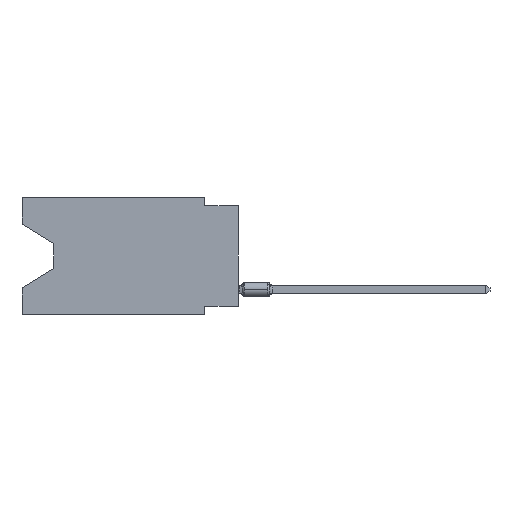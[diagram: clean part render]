
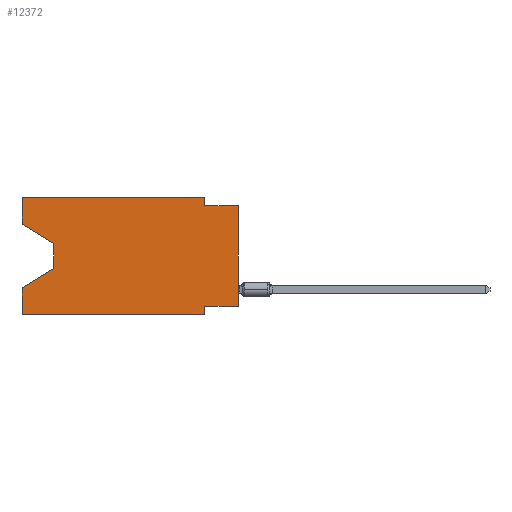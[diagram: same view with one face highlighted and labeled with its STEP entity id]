
A CAD part, left-side view. The second image highlights one B-rep face of the part: STEP entity #12372.
In plain terms, the highlighted planar face has unit normal (-1, 0, 0).
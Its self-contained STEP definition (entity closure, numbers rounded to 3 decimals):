
#201 = VECTOR ( 'NONE', #5137, 1000. ) ;
#222 = AXIS2_PLACEMENT_3D ( 'NONE', #23340, #15614, #23591 ) ;
#711 = ORIENTED_EDGE ( 'NONE', *, *, #15531, .F. ) ;
#891 = ORIENTED_EDGE ( 'NONE', *, *, #18024, .T. ) ;
#923 = CARTESIAN_POINT ( 'NONE',  ( 0., 2.54, 0. ) ) ;
#1017 = VECTOR ( 'NONE', #20075, 1000. ) ;
#1238 = CARTESIAN_POINT ( 'NONE',  ( 0., 16.383, 0. ) ) ;
#1484 = VECTOR ( 'NONE', #4915, 1000. ) ;
#2024 = CARTESIAN_POINT ( 'NONE',  ( 0., 16.383, 0. ) ) ;
#3054 = LINE ( 'NONE', #1238, #4397 ) ;
#3088 = EDGE_CURVE ( 'NONE', #4136, #11339, #17295, .T. ) ;
#3145 = DIRECTION ( 'NONE',  ( 0., 0.855, -0.519 ) ) ;
#3337 = CARTESIAN_POINT ( 'NONE',  ( 0., 13.97, -5.385 ) ) ;
#3357 = LINE ( 'NONE', #13306, #1484 ) ;
#3434 = ORIENTED_EDGE ( 'NONE', *, *, #7880, .F. ) ;
#3718 = EDGE_CURVE ( 'NONE', #4136, #8840, #11868, .T. ) ;
#3720 = CARTESIAN_POINT ( 'NONE',  ( 0., 13.97, -3.505 ) ) ;
#3950 = EDGE_CURVE ( 'NONE', #8452, #16788, #3357, .T. ) ;
#4136 = VERTEX_POINT ( 'NONE', #21675 ) ;
#4397 = VECTOR ( 'NONE', #19028, 1000. ) ;
#4427 = DIRECTION ( 'NONE',  ( 0., -0.855, -0.519 ) ) ;
#4524 = CARTESIAN_POINT ( 'NONE',  ( 0., 16.383, 0. ) ) ;
#4723 = VERTEX_POINT ( 'NONE', #15163 ) ;
#4743 = VECTOR ( 'NONE', #5638, 1000. ) ;
#4868 = VECTOR ( 'NONE', #4427, 1000. ) ;
#4890 = CARTESIAN_POINT ( 'NONE',  ( 0., 0., -0.635 ) ) ;
#4915 = DIRECTION ( 'NONE',  ( 0., 0., -1. ) ) ;
#5137 = DIRECTION ( 'NONE',  ( 0., -1., 0. ) ) ;
#5200 = VECTOR ( 'NONE', #20013, 1000. ) ;
#5401 = FACE_OUTER_BOUND ( 'NONE', #20268, .T. ) ;
#5638 = DIRECTION ( 'NONE',  ( 0., 1., 0. ) ) ;
#6662 = ORIENTED_EDGE ( 'NONE', *, *, #24161, .F. ) ;
#6901 = EDGE_CURVE ( 'NONE', #18964, #8840, #8803, .T. ) ;
#6998 = ORIENTED_EDGE ( 'NONE', *, *, #24707, .F. ) ;
#7002 = VECTOR ( 'NONE', #21537, 1000. ) ;
#7880 = EDGE_CURVE ( 'NONE', #14816, #18964, #18946, .T. ) ;
#8199 = DIRECTION ( 'NONE',  ( 0., 0., -1. ) ) ;
#8452 = VERTEX_POINT ( 'NONE', #3720 ) ;
#8803 = LINE ( 'NONE', #4890, #201 ) ;
#8840 = VERTEX_POINT ( 'NONE', #25519 ) ;
#8968 = VERTEX_POINT ( 'NONE', #10076 ) ;
#10076 = CARTESIAN_POINT ( 'NONE',  ( 0., 16.383, -6.852 ) ) ;
#10216 = ORIENTED_EDGE ( 'NONE', *, *, #3088, .F. ) ;
#10373 = CARTESIAN_POINT ( 'NONE',  ( 0., 16.383, 0. ) ) ;
#10803 = LINE ( 'NONE', #16574, #12685 ) ;
#11339 = VERTEX_POINT ( 'NONE', #22274 ) ;
#11868 = LINE ( 'NONE', #12014, #5200 ) ;
#12014 = CARTESIAN_POINT ( 'NONE',  ( 0., 0., 0. ) ) ;
#12113 = LINE ( 'NONE', #17625, #7002 ) ;
#12372 = ADVANCED_FACE ( 'NONE', ( #5401 ), #23738, .F. ) ;
#12394 = VECTOR ( 'NONE', #3145, 1000. ) ;
#12685 = VECTOR ( 'NONE', #8199, 1000. ) ;
#12788 = ORIENTED_EDGE ( 'NONE', *, *, #25730, .F. ) ;
#13306 = CARTESIAN_POINT ( 'NONE',  ( 0., 13.97, -3.505 ) ) ;
#13551 = ORIENTED_EDGE ( 'NONE', *, *, #14973, .T. ) ;
#14527 = ORIENTED_EDGE ( 'NONE', *, *, #16674, .T. ) ;
#14816 = VERTEX_POINT ( 'NONE', #923 ) ;
#14973 = EDGE_CURVE ( 'NONE', #16788, #8968, #19125, .T. ) ;
#15055 = CARTESIAN_POINT ( 'NONE',  ( 0., 13.97, -5.385 ) ) ;
#15163 = CARTESIAN_POINT ( 'NONE',  ( 0., 16.383, -8.89 ) ) ;
#15531 = EDGE_CURVE ( 'NONE', #11339, #19263, #10803, .T. ) ;
#15614 = DIRECTION ( 'NONE',  ( 1., 0., 0. ) ) ;
#16260 = ORIENTED_EDGE ( 'NONE', *, *, #3718, .T. ) ;
#16574 = CARTESIAN_POINT ( 'NONE',  ( 0., 2.54, -8.89 ) ) ;
#16674 = EDGE_CURVE ( 'NONE', #23670, #8452, #20630, .T. ) ;
#16788 = VERTEX_POINT ( 'NONE', #3337 ) ;
#17295 = LINE ( 'NONE', #21351, #4743 ) ;
#17625 = CARTESIAN_POINT ( 'NONE',  ( 0., 16.383, -8.89 ) ) ;
#18019 = CARTESIAN_POINT ( 'NONE',  ( 0., 2.54, -8.89 ) ) ;
#18024 = EDGE_CURVE ( 'NONE', #4723, #19263, #12113, .T. ) ;
#18239 = LINE ( 'NONE', #2024, #1017 ) ;
#18946 = LINE ( 'NONE', #24976, #25599 ) ;
#18964 = VERTEX_POINT ( 'NONE', #22346 ) ;
#19028 = DIRECTION ( 'NONE',  ( 0., 0., 1. ) ) ;
#19125 = LINE ( 'NONE', #15055, #12394 ) ;
#19263 = VERTEX_POINT ( 'NONE', #18019 ) ;
#19901 = ORIENTED_EDGE ( 'NONE', *, *, #6901, .F. ) ;
#19947 = DIRECTION ( 'NONE',  ( 0., 0., 1. ) ) ;
#20013 = DIRECTION ( 'NONE',  ( 0., 0., 1. ) ) ;
#20075 = DIRECTION ( 'NONE',  ( 0., -1., 0. ) ) ;
#20178 = ORIENTED_EDGE ( 'NONE', *, *, #3950, .T. ) ;
#20190 = LINE ( 'NONE', #10373, #24399 ) ;
#20268 = EDGE_LOOP ( 'NONE', ( #14527, #20178, #13551, #12788, #891, #711, #10216, #16260, #19901, #3434, #6998, #6662 ) ) ;
#20584 = VERTEX_POINT ( 'NONE', #4524 ) ;
#20630 = LINE ( 'NONE', #22347, #4868 ) ;
#21026 = DIRECTION ( 'NONE',  ( 0., 0., -1. ) ) ;
#21174 = CARTESIAN_POINT ( 'NONE',  ( 0., 16.383, -2.038 ) ) ;
#21351 = CARTESIAN_POINT ( 'NONE',  ( 0., 0., -8.255 ) ) ;
#21537 = DIRECTION ( 'NONE',  ( 0., -1., 0. ) ) ;
#21675 = CARTESIAN_POINT ( 'NONE',  ( 0., 0., -8.255 ) ) ;
#22274 = CARTESIAN_POINT ( 'NONE',  ( 0., 2.54, -8.255 ) ) ;
#22346 = CARTESIAN_POINT ( 'NONE',  ( 0., 2.54, -0.635 ) ) ;
#22347 = CARTESIAN_POINT ( 'NONE',  ( 0., 16.383, -2.038 ) ) ;
#23340 = CARTESIAN_POINT ( 'NONE',  ( 0., 16.383, 0. ) ) ;
#23591 = DIRECTION ( 'NONE',  ( 0., 0., -1. ) ) ;
#23670 = VERTEX_POINT ( 'NONE', #21174 ) ;
#23738 = PLANE ( 'NONE',  #222 ) ;
#24161 = EDGE_CURVE ( 'NONE', #23670, #20584, #20190, .T. ) ;
#24399 = VECTOR ( 'NONE', #19947, 1000. ) ;
#24707 = EDGE_CURVE ( 'NONE', #20584, #14816, #18239, .T. ) ;
#24976 = CARTESIAN_POINT ( 'NONE',  ( 0., 2.54, 0. ) ) ;
#25519 = CARTESIAN_POINT ( 'NONE',  ( 0., 0., -0.635 ) ) ;
#25599 = VECTOR ( 'NONE', #21026, 1000. ) ;
#25730 = EDGE_CURVE ( 'NONE', #4723, #8968, #3054, .T. ) ;
